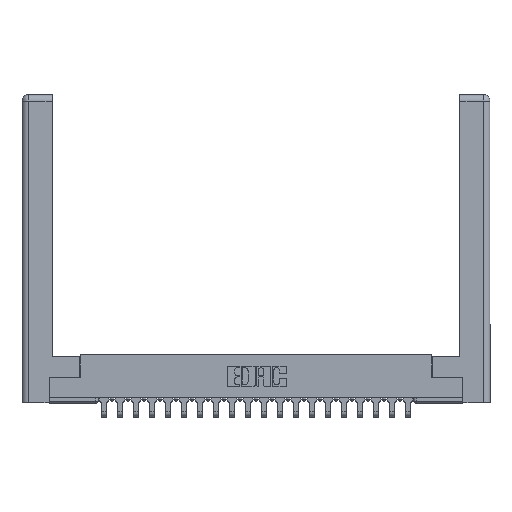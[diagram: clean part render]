
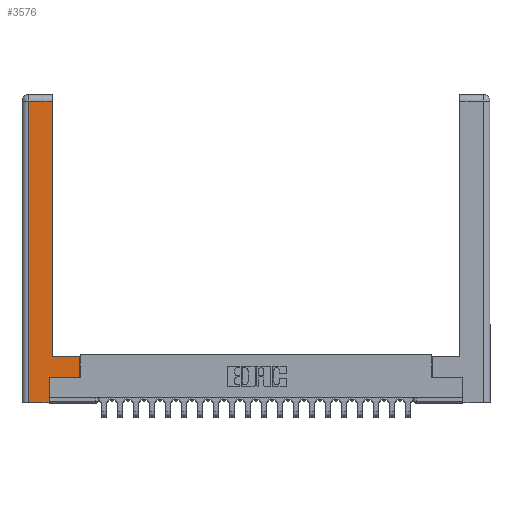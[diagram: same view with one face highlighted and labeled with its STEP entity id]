
A CAD part, top view. The second image highlights one B-rep face of the part: STEP entity #3576.
In plain terms, the highlighted planar face has unit normal (0, 0, 1).
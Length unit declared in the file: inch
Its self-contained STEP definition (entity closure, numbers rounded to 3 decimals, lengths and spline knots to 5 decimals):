
#21 = ORIENTED_EDGE ( 'NONE', *, *, #12494, .T. ) ;
#75 = VECTOR ( 'NONE', #16910, 39.37008 ) ;
#390 = CARTESIAN_POINT ( 'NONE',  ( 0.265, 0., 0. ) ) ;
#494 = LINE ( 'NONE', #7029, #776 ) ;
#776 = VECTOR ( 'NONE', #19230, 39.37008 ) ;
#2062 = LINE ( 'NONE', #14289, #6964 ) ;
#2938 = ORIENTED_EDGE ( 'NONE', *, *, #22019, .T. ) ;
#3171 = CARTESIAN_POINT ( 'NONE',  ( 0., 0., 0. ) ) ;
#3576 = ADVANCED_FACE ( 'NONE', ( #15652 ), #13854, .F. ) ;
#4371 = LINE ( 'NONE', #12086, #18537 ) ;
#4640 = VECTOR ( 'NONE', #11958, 39.37008 ) ;
#4884 = VERTEX_POINT ( 'NONE', #10390 ) ;
#4979 = EDGE_LOOP ( 'NONE', ( #9359, #21, #17688, #17983, #6444, #5612, #7972, #2938 ) ) ;
#5327 = VERTEX_POINT ( 'NONE', #17224 ) ;
#5435 = VERTEX_POINT ( 'NONE', #15789 ) ;
#5612 = ORIENTED_EDGE ( 'NONE', *, *, #19019, .T. ) ;
#6444 = ORIENTED_EDGE ( 'NONE', *, *, #20100, .T. ) ;
#6717 = DIRECTION ( 'NONE',  ( 0., -1., 0. ) ) ;
#6964 = VECTOR ( 'NONE', #15733, 39.37008 ) ;
#7029 = CARTESIAN_POINT ( 'NONE',  ( 0.295, 0.45, 0. ) ) ;
#7806 = VECTOR ( 'NONE', #6717, 39.37008 ) ;
#7972 = ORIENTED_EDGE ( 'NONE', *, *, #15900, .T. ) ;
#8389 = DIRECTION ( 'NONE',  ( 0., 1., 0. ) ) ;
#9359 = ORIENTED_EDGE ( 'NONE', *, *, #19339, .T. ) ;
#10201 = VECTOR ( 'NONE', #18878, 39.37008 ) ;
#10223 = EDGE_CURVE ( 'NONE', #12884, #20800, #21463, .T. ) ;
#10390 = CARTESIAN_POINT ( 'NONE',  ( 0.295, 2.94, 0. ) ) ;
#11752 = VERTEX_POINT ( 'NONE', #18605 ) ;
#11958 = DIRECTION ( 'NONE',  ( 0., 1., 0. ) ) ;
#12086 = CARTESIAN_POINT ( 'NONE',  ( 0.565, 0.245, 0. ) ) ;
#12494 = EDGE_CURVE ( 'NONE', #4884, #12884, #20281, .T. ) ;
#12831 = LINE ( 'NONE', #17150, #21547 ) ;
#12884 = VERTEX_POINT ( 'NONE', #19841 ) ;
#13125 = LINE ( 'NONE', #18865, #4640 ) ;
#13177 = AXIS2_PLACEMENT_3D ( 'NONE', #3171, #13550, #20622 ) ;
#13550 = DIRECTION ( 'NONE',  ( 0., 0., -1. ) ) ;
#13733 = CARTESIAN_POINT ( 'NONE',  ( 0.0615, 2.94, 0. ) ) ;
#13763 = DIRECTION ( 'NONE',  ( 1., 0., 0. ) ) ;
#13854 = PLANE ( 'NONE',  #13177 ) ;
#14289 = CARTESIAN_POINT ( 'NONE',  ( 0.565, 0.45, 0. ) ) ;
#15043 = CARTESIAN_POINT ( 'NONE',  ( 0.265, 0., 0. ) ) ;
#15652 = FACE_OUTER_BOUND ( 'NONE', #4979, .T. ) ;
#15733 = DIRECTION ( 'NONE',  ( 0., 1., 0. ) ) ;
#15789 = CARTESIAN_POINT ( 'NONE',  ( 0.295, 0.45, 0. ) ) ;
#15892 = LINE ( 'NONE', #15043, #75 ) ;
#15900 = EDGE_CURVE ( 'NONE', #5327, #11752, #2062, .T. ) ;
#16649 = VERTEX_POINT ( 'NONE', #19350 ) ;
#16910 = DIRECTION ( 'NONE',  ( 1., 0., 0. ) ) ;
#17150 = CARTESIAN_POINT ( 'NONE',  ( 0.295, 3., 0. ) ) ;
#17162 = CARTESIAN_POINT ( 'NONE',  ( 0.0615, 0., 0. ) ) ;
#17224 = CARTESIAN_POINT ( 'NONE',  ( 0.565, 0.245, 0. ) ) ;
#17688 = ORIENTED_EDGE ( 'NONE', *, *, #10223, .T. ) ;
#17983 = ORIENTED_EDGE ( 'NONE', *, *, #18077, .T. ) ;
#18077 = EDGE_CURVE ( 'NONE', #20800, #18483, #15892, .T. ) ;
#18483 = VERTEX_POINT ( 'NONE', #390 ) ;
#18537 = VECTOR ( 'NONE', #13763, 39.37008 ) ;
#18605 = CARTESIAN_POINT ( 'NONE',  ( 0.565, 0.45, 0. ) ) ;
#18865 = CARTESIAN_POINT ( 'NONE',  ( 0.265, 0.245, 0. ) ) ;
#18878 = DIRECTION ( 'NONE',  ( -1., 0., 0. ) ) ;
#19019 = EDGE_CURVE ( 'NONE', #16649, #5327, #4371, .T. ) ;
#19230 = DIRECTION ( 'NONE',  ( -1., 0., 0. ) ) ;
#19339 = EDGE_CURVE ( 'NONE', #5435, #4884, #12831, .T. ) ;
#19350 = CARTESIAN_POINT ( 'NONE',  ( 0.265, 0.245, 0. ) ) ;
#19841 = CARTESIAN_POINT ( 'NONE',  ( 0.0615, 2.94, 0. ) ) ;
#20100 = EDGE_CURVE ( 'NONE', #18483, #16649, #13125, .T. ) ;
#20281 = LINE ( 'NONE', #13733, #10201 ) ;
#20622 = DIRECTION ( 'NONE',  ( -1., 0., 0. ) ) ;
#20800 = VERTEX_POINT ( 'NONE', #20850 ) ;
#20850 = CARTESIAN_POINT ( 'NONE',  ( 0.0615, 0., 0. ) ) ;
#21463 = LINE ( 'NONE', #17162, #7806 ) ;
#21547 = VECTOR ( 'NONE', #8389, 39.37008 ) ;
#22019 = EDGE_CURVE ( 'NONE', #11752, #5435, #494, .T. ) ;
